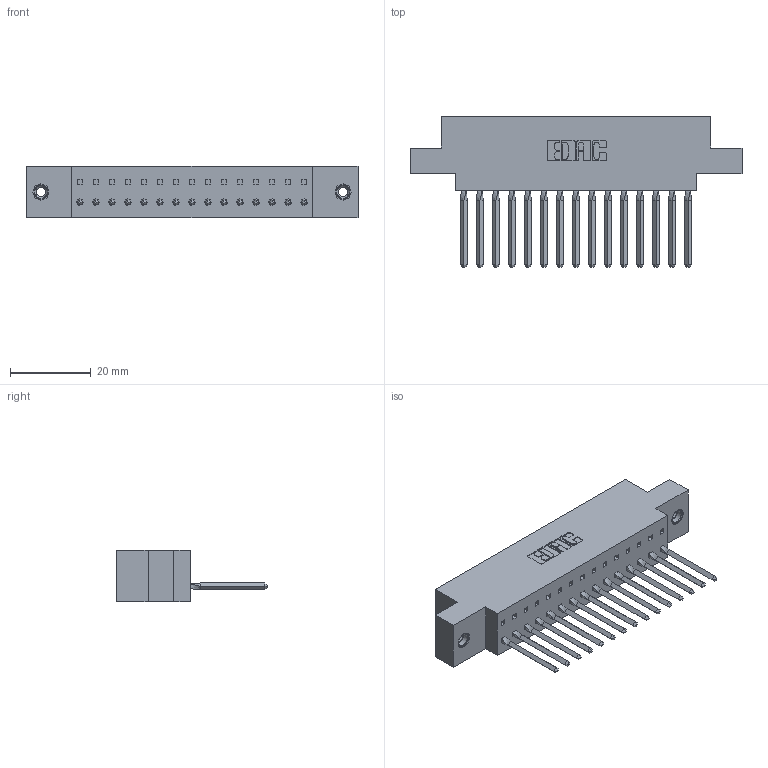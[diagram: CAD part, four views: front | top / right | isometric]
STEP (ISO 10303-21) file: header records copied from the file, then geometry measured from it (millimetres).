
FILE_DESCRIPTION (( 'STEP AP203' ), '1' );
FILE_NAME ('317-015-541-678.STEP', '2020-02-27T15:06:56', ( '' ), ( '' ), 'SwSTEP 2.0', 'SolidWorks 2016', '' );
FILE_SCHEMA (( 'CONFIG_CONTROL_DESIGN' ));
Length unit declared in the file: inch
Products named in the file (4): 317-015-541-678; 345-250-001_345-250-003-102; 317 Part_.156 Dia - TI; 317-290-002_541
Assembly tree (18 placements, depth 2):
  317-015-541-678
    317 Part_.156 Dia - TI
    317-290-002_541  x15
    345-250-001_345-250-003-102  x2
Bounding box: 82.14 x 37.34 x 12.7 mm (x, y, z)
Volume: 12484.2 mm3; surface area: 16762.4 mm2
Topology: 18 solids, 18 shells, 2442 faces, 6921 edges, 4496 vertices
Faces by surface type: plane 1950, cylinder 416, bspline 60, cone 12, torus 4
Entity records: 27703 total; most frequent: CARTESIAN_POINT 5521, ORIENTED_EDGE 4782, DIRECTION 3951, EDGE_CURVE 2391, LINE 2007, VECTOR 2007, VERTEX_POINT 1582, AXIS2_PLACEMENT_3D 972
